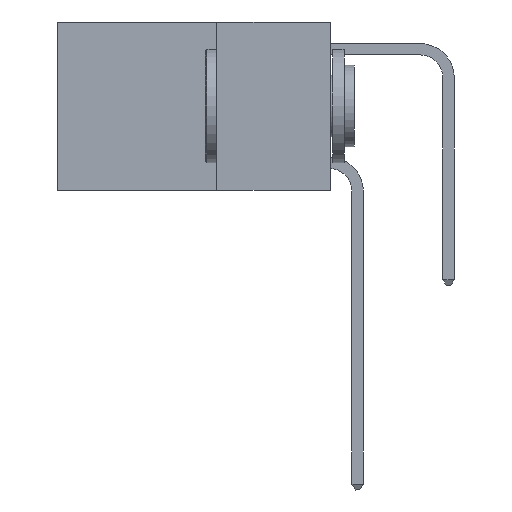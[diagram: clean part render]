
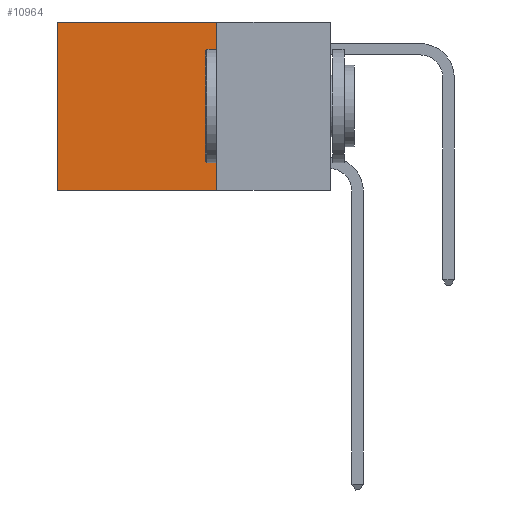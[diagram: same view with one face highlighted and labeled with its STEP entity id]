
A CAD part, left-side view. The second image highlights one B-rep face of the part: STEP entity #10964.
In plain terms, the highlighted planar face has unit normal (-1, 0, 0).
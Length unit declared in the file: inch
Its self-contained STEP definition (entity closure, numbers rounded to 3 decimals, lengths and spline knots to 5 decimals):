
#14 = EDGE_CURVE ( 'NONE', #1787, #2399, #1721, .T. ) ;
#790 = CARTESIAN_POINT ( 'NONE',  ( 0.2625, 0.6, -0.37 ) ) ;
#1024 = CARTESIAN_POINT ( 'NONE',  ( 0.2625, 0.25, 0. ) ) ;
#1132 = DIRECTION ( 'NONE',  ( 0., 0., -1. ) ) ;
#1256 = EDGE_CURVE ( 'NONE', #9653, #4664, #7815, .T. ) ;
#1721 = LINE ( 'NONE', #5150, #10874 ) ;
#1787 = VERTEX_POINT ( 'NONE', #6498 ) ;
#2129 = LINE ( 'NONE', #3270, #6866 ) ;
#2206 = EDGE_CURVE ( 'NONE', #1787, #9653, #8073, .T. ) ;
#2283 = CARTESIAN_POINT ( 'NONE',  ( 0.2625, 0.25, 0. ) ) ;
#2399 = VERTEX_POINT ( 'NONE', #9067 ) ;
#3175 = DIRECTION ( 'NONE',  ( 0., 0., -1. ) ) ;
#3270 = CARTESIAN_POINT ( 'NONE',  ( 0.2625, 0.6, 0. ) ) ;
#3856 = FACE_OUTER_BOUND ( 'NONE', #7258, .T. ) ;
#3989 = ORIENTED_EDGE ( 'NONE', *, *, #14, .T. ) ;
#4222 = ORIENTED_EDGE ( 'NONE', *, *, #2206, .F. ) ;
#4340 = ORIENTED_EDGE ( 'NONE', *, *, #8091, .T. ) ;
#4482 = CARTESIAN_POINT ( 'NONE',  ( 0.2625, 0.25, -0.37 ) ) ;
#4664 = VERTEX_POINT ( 'NONE', #790 ) ;
#4981 = DIRECTION ( 'NONE',  ( 0., 0., -1. ) ) ;
#5150 = CARTESIAN_POINT ( 'NONE',  ( 0.2625, 0.25, 0. ) ) ;
#5186 = ORIENTED_EDGE ( 'NONE', *, *, #1256, .F. ) ;
#6464 = AXIS2_PLACEMENT_3D ( 'NONE', #2283, #8496, #3175 ) ;
#6498 = CARTESIAN_POINT ( 'NONE',  ( 0.2625, 0.25, 0. ) ) ;
#6866 = VECTOR ( 'NONE', #4981, 39.37008 ) ;
#7258 = EDGE_LOOP ( 'NONE', ( #4340, #5186, #4222, #3989 ) ) ;
#7611 = PLANE ( 'NONE',  #6464 ) ;
#7815 = LINE ( 'NONE', #4482, #10189 ) ;
#8073 = LINE ( 'NONE', #1024, #10691 ) ;
#8091 = EDGE_CURVE ( 'NONE', #2399, #4664, #2129, .T. ) ;
#8496 = DIRECTION ( 'NONE',  ( 1., 0., 0. ) ) ;
#9067 = CARTESIAN_POINT ( 'NONE',  ( 0.2625, 0.6, 0. ) ) ;
#9653 = VERTEX_POINT ( 'NONE', #10108 ) ;
#10108 = CARTESIAN_POINT ( 'NONE',  ( 0.2625, 0.25, -0.37 ) ) ;
#10189 = VECTOR ( 'NONE', #10662, 39.37008 ) ;
#10662 = DIRECTION ( 'NONE',  ( 0., 1., 0. ) ) ;
#10691 = VECTOR ( 'NONE', #1132, 39.37008 ) ;
#10874 = VECTOR ( 'NONE', #10908, 39.37008 ) ;
#10908 = DIRECTION ( 'NONE',  ( 0., 1., 0. ) ) ;
#10964 = ADVANCED_FACE ( 'NONE', ( #3856 ), #7611, .F. ) ;
